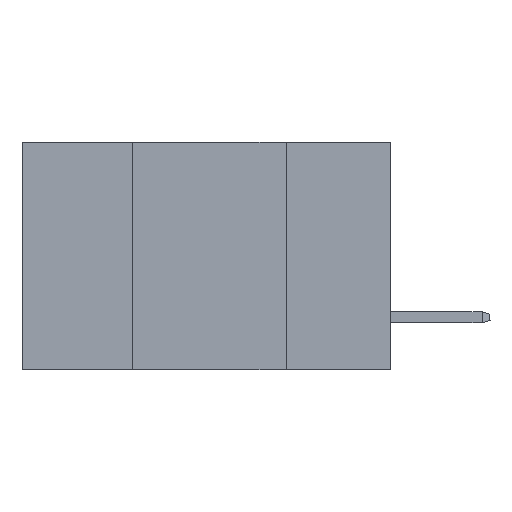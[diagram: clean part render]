
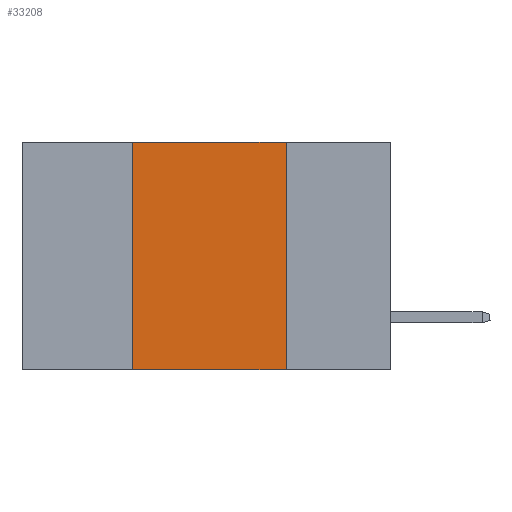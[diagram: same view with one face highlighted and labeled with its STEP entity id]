
A CAD part, left-side view. The second image highlights one B-rep face of the part: STEP entity #33208.
In plain terms, the highlighted planar face has unit normal (-1, 0, 0).
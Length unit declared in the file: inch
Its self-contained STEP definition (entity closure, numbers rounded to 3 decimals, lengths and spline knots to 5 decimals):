
#1163 = DIRECTION ( 'NONE',  ( 0., 0., -1. ) ) ;
#1996 = ORIENTED_EDGE ( 'NONE', *, *, #8742, .F. ) ;
#2304 = VECTOR ( 'NONE', #23819, 39.37008 ) ;
#6563 = LINE ( 'NONE', #43888, #41783 ) ;
#7325 = DIRECTION ( 'NONE',  ( 0., -1., 0. ) ) ;
#8742 = EDGE_CURVE ( 'NONE', #14668, #40886, #12004, .T. ) ;
#12004 = LINE ( 'NONE', #31650, #2304 ) ;
#14314 = CARTESIAN_POINT ( 'NONE',  ( 0., 0.17, -0.37 ) ) ;
#14668 = VERTEX_POINT ( 'NONE', #19722 ) ;
#14950 = DIRECTION ( 'NONE',  ( 0., 0., -1. ) ) ;
#19434 = CARTESIAN_POINT ( 'NONE',  ( 0., 0.17, 0. ) ) ;
#19722 = CARTESIAN_POINT ( 'NONE',  ( 0., 0.42, -0.37 ) ) ;
#21200 = EDGE_CURVE ( 'NONE', #14668, #27837, #38816, .T. ) ;
#21936 = CARTESIAN_POINT ( 'NONE',  ( 0., 0.42, 0. ) ) ;
#22807 = ORIENTED_EDGE ( 'NONE', *, *, #38888, .F. ) ;
#23211 = LINE ( 'NONE', #19434, #45842 ) ;
#23819 = DIRECTION ( 'NONE',  ( 0., 0., 1. ) ) ;
#24155 = DIRECTION ( 'NONE',  ( 0., -1., 0. ) ) ;
#27268 = EDGE_LOOP ( 'NONE', ( #22807, #28822, #1996, #40789 ) ) ;
#27657 = AXIS2_PLACEMENT_3D ( 'NONE', #36732, #37184, #14950 ) ;
#27837 = VERTEX_POINT ( 'NONE', #14314 ) ;
#28385 = CARTESIAN_POINT ( 'NONE',  ( 0., 0.6, -0.37 ) ) ;
#28822 = ORIENTED_EDGE ( 'NONE', *, *, #34673, .F. ) ;
#29204 = FACE_OUTER_BOUND ( 'NONE', #27268, .T. ) ;
#31650 = CARTESIAN_POINT ( 'NONE',  ( 0., 0.42, 0. ) ) ;
#33021 = PLANE ( 'NONE',  #27657 ) ;
#33208 = ADVANCED_FACE ( 'NONE', ( #29204 ), #33021, .F. ) ;
#34673 = EDGE_CURVE ( 'NONE', #40886, #41304, #6563, .T. ) ;
#36732 = CARTESIAN_POINT ( 'NONE',  ( 0., 0.6, 0. ) ) ;
#37184 = DIRECTION ( 'NONE',  ( 1., 0., 0. ) ) ;
#38816 = LINE ( 'NONE', #28385, #42263 ) ;
#38888 = EDGE_CURVE ( 'NONE', #41304, #27837, #23211, .T. ) ;
#40789 = ORIENTED_EDGE ( 'NONE', *, *, #21200, .T. ) ;
#40886 = VERTEX_POINT ( 'NONE', #21936 ) ;
#41304 = VERTEX_POINT ( 'NONE', #47063 ) ;
#41783 = VECTOR ( 'NONE', #7325, 39.37008 ) ;
#42263 = VECTOR ( 'NONE', #24155, 39.37008 ) ;
#43888 = CARTESIAN_POINT ( 'NONE',  ( 0., 0.6, 0. ) ) ;
#45842 = VECTOR ( 'NONE', #1163, 39.37008 ) ;
#47063 = CARTESIAN_POINT ( 'NONE',  ( 0., 0.17, 0. ) ) ;
